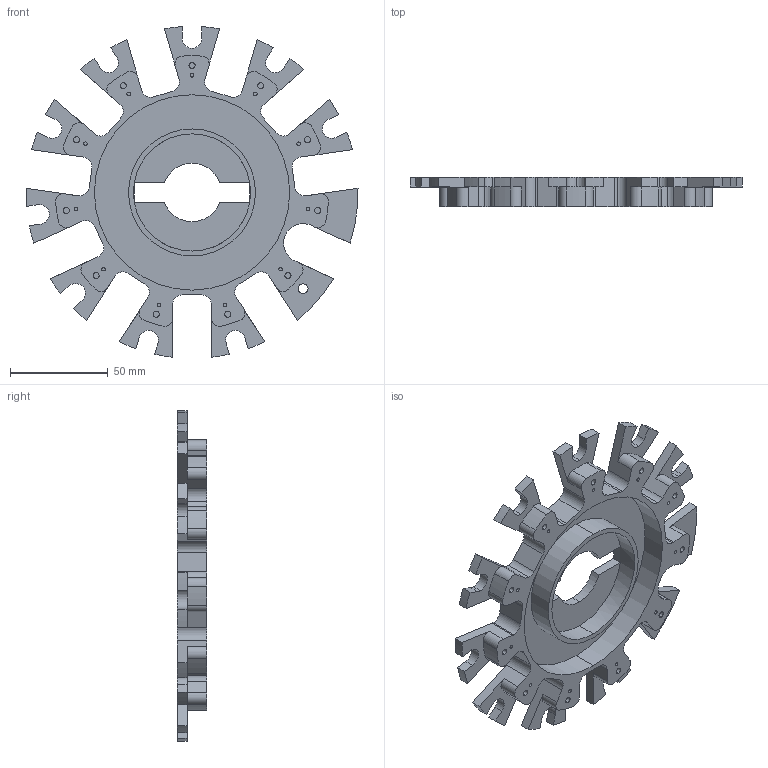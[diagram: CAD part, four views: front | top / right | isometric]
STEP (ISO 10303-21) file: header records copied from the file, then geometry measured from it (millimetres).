
FILE_DESCRIPTION (( 'STEP AP214' ), '1' );
FILE_NAME ('spindle-front half.STEP', '2013-12-23T14:49:58', ( '' ), ( '' ), 'SwSTEP 2.0', 'SolidWorks 2013', '' );
FILE_SCHEMA (( 'AUTOMOTIVE_DESIGN' ));
Length unit declared in the file: millimetre
Products named in the file (1): spindle-front half
Bounding box: 169.97 x 15 x 169.26 mm (x, y, z)
Volume: 99236.5 mm3; surface area: 52266.2 mm2
Topology: 1 solids, 1 shells, 248 faces, 666 edges, 444 vertices
Faces by surface type: cylinder 155, plane 93
Entity records: 7946 total; most frequent: DIRECTION 1478, CARTESIAN_POINT 1359, ORIENTED_EDGE 1332, EDGE_CURVE 666, AXIS2_PLACEMENT_3D 563, VERTEX_POINT 444, VECTOR 352, LINE 352
